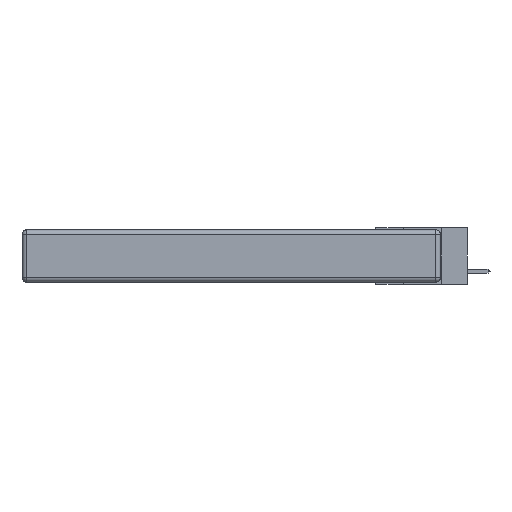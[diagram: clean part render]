
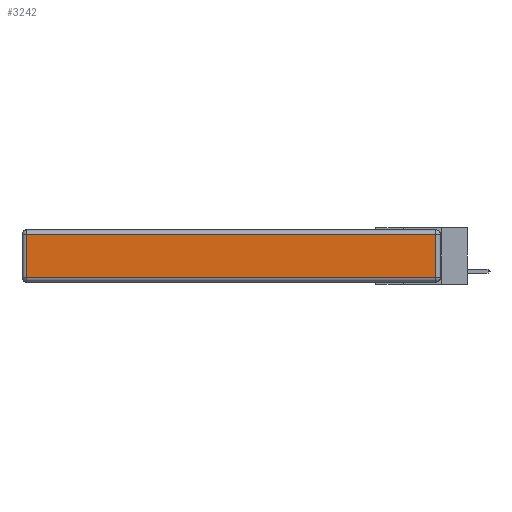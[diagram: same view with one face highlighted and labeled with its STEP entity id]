
A CAD part, left-side view. The second image highlights one B-rep face of the part: STEP entity #3242.
In plain terms, the highlighted planar face has unit normal (-1, 0, 0).
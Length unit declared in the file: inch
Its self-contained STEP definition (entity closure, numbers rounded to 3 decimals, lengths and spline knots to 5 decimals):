
#626 = VECTOR ( 'NONE', #6267, 39.37008 ) ;
#677 = VECTOR ( 'NONE', #20522, 39.37008 ) ;
#1685 = VECTOR ( 'NONE', #12520, 39.37008 ) ;
#3028 = ORIENTED_EDGE ( 'NONE', *, *, #9701, .T. ) ;
#3242 = ADVANCED_FACE ( 'NONE', ( #21254 ), #6272, .T. ) ;
#3393 = CARTESIAN_POINT ( 'NONE',  ( 0., 2.72, -0.313 ) ) ;
#3488 = ORIENTED_EDGE ( 'NONE', *, *, #5026, .T. ) ;
#4129 = CARTESIAN_POINT ( 'NONE',  ( 0., 0.03, -0.313 ) ) ;
#4398 = DIRECTION ( 'NONE',  ( 0., 1., 0. ) ) ;
#5026 = EDGE_CURVE ( 'NONE', #12925, #8703, #11268, .T. ) ;
#5496 = CARTESIAN_POINT ( 'NONE',  ( 0., 0.03, -0.343 ) ) ;
#6267 = DIRECTION ( 'NONE',  ( 0., 0., 1. ) ) ;
#6272 = PLANE ( 'NONE',  #18072 ) ;
#6607 = DIRECTION ( 'NONE',  ( 0., 0., 1. ) ) ;
#8236 = ORIENTED_EDGE ( 'NONE', *, *, #13178, .T. ) ;
#8703 = VERTEX_POINT ( 'NONE', #20771 ) ;
#9701 = EDGE_CURVE ( 'NONE', #8703, #10988, #19446, .T. ) ;
#9875 = VERTEX_POINT ( 'NONE', #4129 ) ;
#10134 = CARTESIAN_POINT ( 'NONE',  ( 0., 0., -0.343 ) ) ;
#10660 = VECTOR ( 'NONE', #4398, 39.37008 ) ;
#10988 = VERTEX_POINT ( 'NONE', #3393 ) ;
#11268 = LINE ( 'NONE', #14340, #10660 ) ;
#12520 = DIRECTION ( 'NONE',  ( 0., 0., -1. ) ) ;
#12925 = VERTEX_POINT ( 'NONE', #20706 ) ;
#13178 = EDGE_CURVE ( 'NONE', #9875, #12925, #18102, .T. ) ;
#14340 = CARTESIAN_POINT ( 'NONE',  ( 0., 2.75, -0.03 ) ) ;
#15030 = EDGE_LOOP ( 'NONE', ( #17794, #8236, #3488, #3028 ) ) ;
#15940 = DIRECTION ( 'NONE',  ( -1., 0., 0. ) ) ;
#16581 = CARTESIAN_POINT ( 'NONE',  ( 0., 0., -0.313 ) ) ;
#17545 = LINE ( 'NONE', #16581, #677 ) ;
#17794 = ORIENTED_EDGE ( 'NONE', *, *, #22635, .T. ) ;
#18072 = AXIS2_PLACEMENT_3D ( 'NONE', #10134, #15940, #6607 ) ;
#18102 = LINE ( 'NONE', #5496, #626 ) ;
#19446 = LINE ( 'NONE', #22084, #1685 ) ;
#20522 = DIRECTION ( 'NONE',  ( 0., -1., 0. ) ) ;
#20706 = CARTESIAN_POINT ( 'NONE',  ( 0., 0.03, -0.03 ) ) ;
#20771 = CARTESIAN_POINT ( 'NONE',  ( 0., 2.72, -0.03 ) ) ;
#21254 = FACE_OUTER_BOUND ( 'NONE', #15030, .T. ) ;
#22084 = CARTESIAN_POINT ( 'NONE',  ( 0., 2.72, -0.343 ) ) ;
#22635 = EDGE_CURVE ( 'NONE', #10988, #9875, #17545, .T. ) ;
